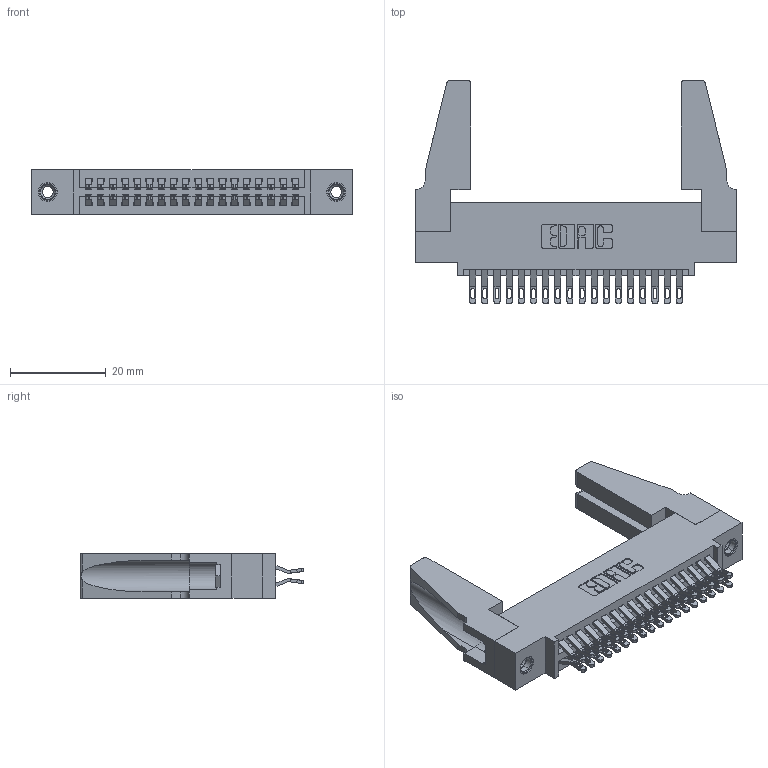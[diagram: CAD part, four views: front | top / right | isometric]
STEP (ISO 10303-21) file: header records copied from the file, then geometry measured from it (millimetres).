
FILE_DESCRIPTION (( 'STEP AP203' ), '1' );
FILE_NAME ('345-036-555-588.STEP', '2019-10-28T12:39:16', ( '' ), ( '' ), 'SwSTEP 2.0', 'SolidWorks 2016', '' );
FILE_SCHEMA (( 'CONFIG_CONTROL_DESIGN' ));
Length unit declared in the file: inch
Products named in the file (5): 345-250-001_345-250-001-102; 345-220-078_345-220-088; 345-036-555-588; 345 Part_0.110 Offset - 0.156 Dia-TH; 345-292-001_555 Tail
Assembly tree (41 placements, depth 2):
  345-036-555-588
    345 Part_0.110 Offset - 0.156 Dia-TH
    345-292-001_555 Tail  x36
    345-250-001_345-250-001-102  x2
    345-220-078_345-220-088  x2
Bounding box: 66.95 x 46.79 x 9.4 mm (x, y, z)
Volume: 9564.7 mm3; surface area: 12443.9 mm2
Topology: 41 solids, 41 shells, 2270 faces, 7039 edges, 4682 vertices
Faces by surface type: plane 1272, cylinder 982, cone 12, torus 4
Entity records: 19960 total; most frequent: CARTESIAN_POINT 3400, ORIENTED_EDGE 3264, DIRECTION 3000, EDGE_CURVE 1632, LINE 1366, VECTOR 1366, VERTEX_POINT 1082, AXIS2_PLACEMENT_3D 817
